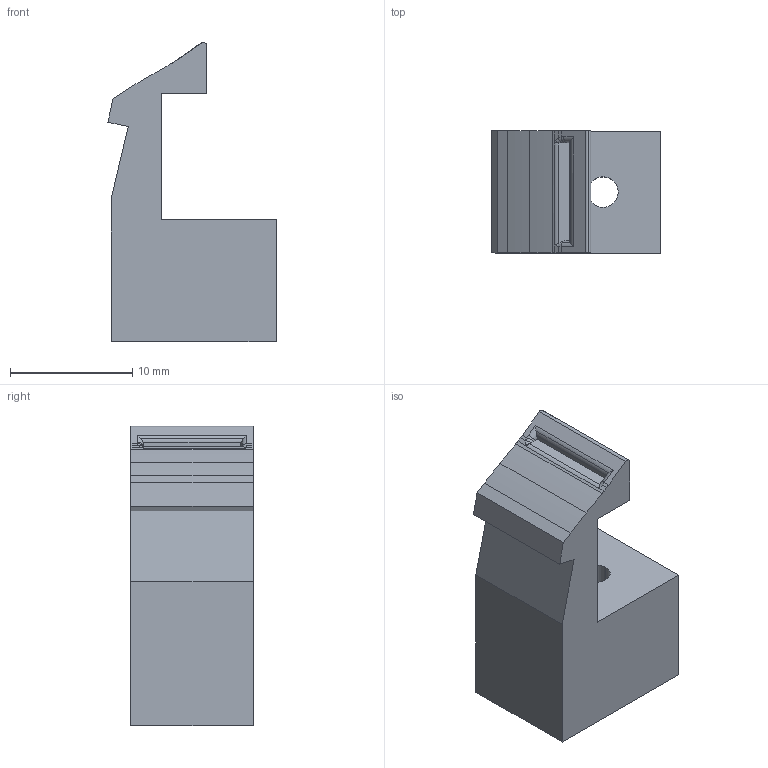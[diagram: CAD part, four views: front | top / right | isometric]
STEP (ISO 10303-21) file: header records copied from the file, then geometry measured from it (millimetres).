
FILE_DESCRIPTION(('STEP AP214'),'1');
FILE_NAME('WTF9E Feed Ramp.stl.stp','2020-09-01T22:09:45',(' '),(' '),'Spatial InterOp 3D',' ',' ');
FILE_SCHEMA(('AUTOMOTIVE_DESIGN { 1 0 10303 214 1 1 1 1 }'));
Length unit declared in the file: metre
Products named in the file (1): Solid
Bounding box: 13.79 x 10 x 24.53 mm (x, y, z)
Volume: 1826.7 mm3; surface area: 1264.5 mm2
Topology: 1 solids, 1 shells, 41 faces, 112 edges, 72 vertices
Faces by surface type: plane 18, cylinder 17, bspline 6
Entity records: 2215 total; most frequent: CARTESIAN_POINT 1172, ORIENTED_EDGE 222, DIRECTION 198, EDGE_CURVE 111, VERTEX_POINT 72, AXIS2_PLACEMENT_3D 66, LINE 66, VECTOR 66
